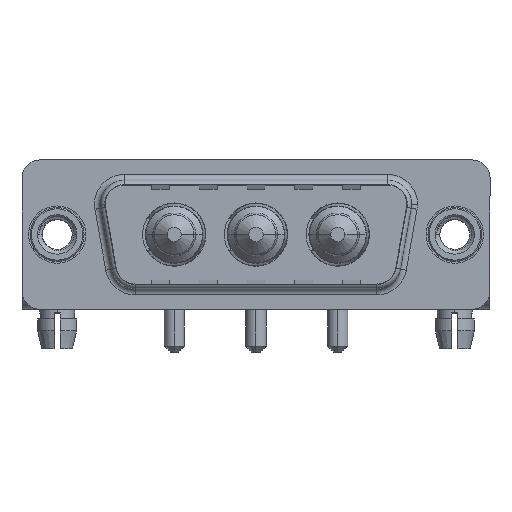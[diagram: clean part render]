
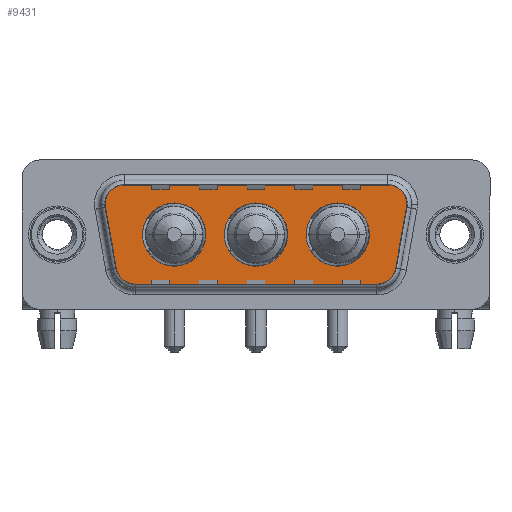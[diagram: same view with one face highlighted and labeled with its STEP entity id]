
A CAD part, top view. The second image highlights one B-rep face of the part: STEP entity #9431.
In plain terms, the highlighted planar face has unit normal (0, 0, 1).
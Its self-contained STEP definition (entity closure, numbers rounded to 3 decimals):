
#274 = VERTEX_POINT ( 'NONE', #9178 ) ;
#331 = FACE_BOUND ( 'NONE', #2962, .T. ) ;
#351 = EDGE_CURVE ( 'NONE', #10542, #8875, #3159, .T. ) ;
#378 = VERTEX_POINT ( 'NONE', #1753 ) ;
#496 = FACE_OUTER_BOUND ( 'NONE', #13904, .T. ) ;
#556 = CARTESIAN_POINT ( 'NONE',  ( 9.8, 0., 0. ) ) ;
#640 = CARTESIAN_POINT ( 'NONE',  ( 20.85, 0., 0. ) ) ;
#768 = ORIENTED_EDGE ( 'NONE', *, *, #11275, .T. ) ;
#896 = VERTEX_POINT ( 'NONE', #9669 ) ;
#897 = CARTESIAN_POINT ( 'NONE',  ( 3.441, 2.553, 0. ) ) ;
#939 = VERTEX_POINT ( 'NONE', #15259 ) ;
#1233 = VERTEX_POINT ( 'NONE', #13340 ) ;
#1234 = DIRECTION ( 'NONE',  ( 0., 0., 1. ) ) ;
#1381 = DIRECTION ( 'NONE',  ( -1., 0., 0. ) ) ;
#1605 = DIRECTION ( 'NONE',  ( 0., 0., 1. ) ) ;
#1616 = VECTOR ( 'NONE', #13439, 1000. ) ;
#1753 = CARTESIAN_POINT ( 'NONE',  ( 14., 0., 0. ) ) ;
#1831 = CARTESIAN_POINT ( 'NONE',  ( 23.5, 0., 0. ) ) ;
#1839 = DIRECTION ( 'NONE',  ( 0., 0., 1. ) ) ;
#1972 = CARTESIAN_POINT ( 'NONE',  ( 29.889, 2.9, 0. ) ) ;
#2001 = DIRECTION ( 'NONE',  ( -1., 0., 0. ) ) ;
#2114 = EDGE_CURVE ( 'NONE', #2596, #12028, #15450, .T. ) ;
#2161 = EDGE_LOOP ( 'NONE', ( #13981, #5495 ) ) ;
#2352 = DIRECTION ( 'NONE',  ( 1., 0., 0. ) ) ;
#2442 = CARTESIAN_POINT ( 'NONE',  ( 26.866, -4.9, 0. ) ) ;
#2596 = VERTEX_POINT ( 'NONE', #3486 ) ;
#2664 = DIRECTION ( 'NONE',  ( 0., 0., 1. ) ) ;
#2779 = ORIENTED_EDGE ( 'NONE', *, *, #13818, .F. ) ;
#2815 = FACE_BOUND ( 'NONE', #14606, .T. ) ;
#2962 = EDGE_LOOP ( 'NONE', ( #2779, #12236 ) ) ;
#2989 = CARTESIAN_POINT ( 'NONE',  ( 6.434, -4.9, 0. ) ) ;
#2990 = PLANE ( 'NONE',  #14527 ) ;
#3159 = CIRCLE ( 'NONE', #12820, 2.65 ) ;
#3203 = CARTESIAN_POINT ( 'NONE',  ( 27.889, 2.9, 0. ) ) ;
#3245 = CARTESIAN_POINT ( 'NONE',  ( 26.15, 0., 0. ) ) ;
#3306 = VERTEX_POINT ( 'NONE', #2442 ) ;
#3486 = CARTESIAN_POINT ( 'NONE',  ( 27.889, 4.9, 0. ) ) ;
#3535 = CIRCLE ( 'NONE', #10712, 2.65 ) ;
#3571 = DIRECTION ( 'NONE',  ( 1., 0., 0. ) ) ;
#3762 = CARTESIAN_POINT ( 'NONE',  ( 27.889, 2.9, 0. ) ) ;
#4209 = EDGE_CURVE ( 'NONE', #5974, #2596, #5596, .T. ) ;
#4340 = DIRECTION ( 'NONE',  ( 0., 0., 1. ) ) ;
#4402 = CARTESIAN_POINT ( 'NONE',  ( 12.45, 0., 0. ) ) ;
#4626 = EDGE_CURVE ( 'NONE', #378, #11603, #3535, .T. ) ;
#4787 = ORIENTED_EDGE ( 'NONE', *, *, #12151, .F. ) ;
#4800 = AXIS2_PLACEMENT_3D ( 'NONE', #3203, #1839, #2001 ) ;
#4841 = CIRCLE ( 'NONE', #7334, 2. ) ;
#5003 = LINE ( 'NONE', #897, #9470 ) ;
#5089 = CIRCLE ( 'NONE', #7308, 2.65 ) ;
#5100 = VERTEX_POINT ( 'NONE', #640 ) ;
#5268 = CARTESIAN_POINT ( 'NONE',  ( 16.65, 0., 0. ) ) ;
#5425 = ORIENTED_EDGE ( 'NONE', *, *, #4209, .T. ) ;
#5495 = ORIENTED_EDGE ( 'NONE', *, *, #8730, .F. ) ;
#5596 = CIRCLE ( 'NONE', #6151, 2. ) ;
#5646 = LINE ( 'NONE', #14955, #1616 ) ;
#5895 = CIRCLE ( 'NONE', #4800, 2. ) ;
#5974 = VERTEX_POINT ( 'NONE', #1972 ) ;
#6046 = DIRECTION ( 'NONE',  ( 1., 0., 0. ) ) ;
#6151 = AXIS2_PLACEMENT_3D ( 'NONE', #3762, #9035, #7483 ) ;
#6349 = EDGE_CURVE ( 'NONE', #1233, #3306, #10924, .T. ) ;
#6575 = CARTESIAN_POINT ( 'NONE',  ( 23.5, 0., 0. ) ) ;
#7308 = AXIS2_PLACEMENT_3D ( 'NONE', #1831, #12426, #6046 ) ;
#7334 = AXIS2_PLACEMENT_3D ( 'NONE', #10989, #4340, #1381 ) ;
#7359 = DIRECTION ( 'NONE',  ( -1., 0., 0. ) ) ;
#7436 = CARTESIAN_POINT ( 'NONE',  ( 5.411, 4.9, 0. ) ) ;
#7476 = CARTESIAN_POINT ( 'NONE',  ( 7.15, 0., 0. ) ) ;
#7483 = DIRECTION ( 'NONE',  ( -1., 0., 0. ) ) ;
#7925 = DIRECTION ( 'NONE',  ( 1., 0., 0. ) ) ;
#7970 = ORIENTED_EDGE ( 'NONE', *, *, #13523, .T. ) ;
#8233 = DIRECTION ( 'NONE',  ( 1., 0., 0. ) ) ;
#8308 = DIRECTION ( 'NONE',  ( 0., 0., 1. ) ) ;
#8381 = ORIENTED_EDGE ( 'NONE', *, *, #14727, .T. ) ;
#8510 = CIRCLE ( 'NONE', #9067, 2.65 ) ;
#8730 = EDGE_CURVE ( 'NONE', #8875, #10542, #8510, .T. ) ;
#8859 = ORIENTED_EDGE ( 'NONE', *, *, #2114, .T. ) ;
#8875 = VERTEX_POINT ( 'NONE', #7476 ) ;
#9035 = DIRECTION ( 'NONE',  ( 0., 0., 1. ) ) ;
#9067 = AXIS2_PLACEMENT_3D ( 'NONE', #14460, #2664, #7925 ) ;
#9178 = CARTESIAN_POINT ( 'NONE',  ( 3.441, 2.553, 0. ) ) ;
#9334 = VERTEX_POINT ( 'NONE', #15751 ) ;
#9413 = EDGE_CURVE ( 'NONE', #9334, #939, #5646, .T. ) ;
#9431 = ADVANCED_FACE ( 'NONE', ( #331, #2815, #10835, #496 ), #2990, .T. ) ;
#9470 = VECTOR ( 'NONE', #15270, 1000. ) ;
#9669 = CARTESIAN_POINT ( 'NONE',  ( 4.464, -3.247, 0. ) ) ;
#9840 = EDGE_CURVE ( 'NONE', #3306, #9334, #11967, .T. ) ;
#9943 = CARTESIAN_POINT ( 'NONE',  ( 5.411, 4.9, 0. ) ) ;
#10532 = EDGE_CURVE ( 'NONE', #12929, #5100, #5089, .T. ) ;
#10542 = VERTEX_POINT ( 'NONE', #4402 ) ;
#10658 = AXIS2_PLACEMENT_3D ( 'NONE', #6575, #12949, #14306 ) ;
#10677 = DIRECTION ( 'NONE',  ( 0., 0., 1. ) ) ;
#10712 = AXIS2_PLACEMENT_3D ( 'NONE', #12813, #14169, #3571 ) ;
#10757 = DIRECTION ( 'NONE',  ( 1., 0., 0. ) ) ;
#10835 = FACE_BOUND ( 'NONE', #2161, .T. ) ;
#10874 = AXIS2_PLACEMENT_3D ( 'NONE', #15986, #1605, #8233 ) ;
#10924 = LINE ( 'NONE', #2989, #14618 ) ;
#10989 = CARTESIAN_POINT ( 'NONE',  ( 6.434, -2.9, 0. ) ) ;
#11020 = ORIENTED_EDGE ( 'NONE', *, *, #6349, .T. ) ;
#11149 = AXIS2_PLACEMENT_3D ( 'NONE', #11643, #11561, #2352 ) ;
#11247 = VECTOR ( 'NONE', #7359, 1000. ) ;
#11275 = EDGE_CURVE ( 'NONE', #896, #1233, #4841, .T. ) ;
#11561 = DIRECTION ( 'NONE',  ( 0., 0., 1. ) ) ;
#11572 = ORIENTED_EDGE ( 'NONE', *, *, #9413, .T. ) ;
#11603 = VERTEX_POINT ( 'NONE', #16918 ) ;
#11643 = CARTESIAN_POINT ( 'NONE',  ( 5.411, 2.9, 0. ) ) ;
#11967 = CIRCLE ( 'NONE', #10874, 2. ) ;
#12028 = VERTEX_POINT ( 'NONE', #7436 ) ;
#12151 = EDGE_CURVE ( 'NONE', #5100, #12929, #13677, .T. ) ;
#12186 = DIRECTION ( 'NONE',  ( 1., 0., 0. ) ) ;
#12236 = ORIENTED_EDGE ( 'NONE', *, *, #4626, .F. ) ;
#12426 = DIRECTION ( 'NONE',  ( 0., 0., 1. ) ) ;
#12801 = CIRCLE ( 'NONE', #15529, 2.65 ) ;
#12813 = CARTESIAN_POINT ( 'NONE',  ( 16.65, 0., 0. ) ) ;
#12820 = AXIS2_PLACEMENT_3D ( 'NONE', #556, #8308, #12186 ) ;
#12929 = VERTEX_POINT ( 'NONE', #3245 ) ;
#12949 = DIRECTION ( 'NONE',  ( 0., 0., 1. ) ) ;
#13340 = CARTESIAN_POINT ( 'NONE',  ( 6.434, -4.9, 0. ) ) ;
#13345 = CARTESIAN_POINT ( 'NONE',  ( 26.866, -2.9, 0. ) ) ;
#13439 = DIRECTION ( 'NONE',  ( 0.174, 0.985, 0. ) ) ;
#13523 = EDGE_CURVE ( 'NONE', #274, #896, #5003, .T. ) ;
#13677 = CIRCLE ( 'NONE', #10658, 2.65 ) ;
#13818 = EDGE_CURVE ( 'NONE', #11603, #378, #12801, .T. ) ;
#13904 = EDGE_LOOP ( 'NONE', ( #16893, #11572, #8381, #5425, #8859, #16036, #7970, #768, #11020 ) ) ;
#13981 = ORIENTED_EDGE ( 'NONE', *, *, #351, .F. ) ;
#14169 = DIRECTION ( 'NONE',  ( 0., 0., 1. ) ) ;
#14306 = DIRECTION ( 'NONE',  ( 1., 0., 0. ) ) ;
#14460 = CARTESIAN_POINT ( 'NONE',  ( 9.8, 0., 0. ) ) ;
#14527 = AXIS2_PLACEMENT_3D ( 'NONE', #13345, #10677, #10757 ) ;
#14606 = EDGE_LOOP ( 'NONE', ( #16773, #4787 ) ) ;
#14618 = VECTOR ( 'NONE', #14871, 1000. ) ;
#14727 = EDGE_CURVE ( 'NONE', #939, #5974, #5895, .T. ) ;
#14871 = DIRECTION ( 'NONE',  ( 1., 0., 0. ) ) ;
#14888 = EDGE_CURVE ( 'NONE', #12028, #274, #16372, .T. ) ;
#14955 = CARTESIAN_POINT ( 'NONE',  ( 29.859, 2.553, 0. ) ) ;
#15259 = CARTESIAN_POINT ( 'NONE',  ( 29.859, 2.553, 0. ) ) ;
#15270 = DIRECTION ( 'NONE',  ( 0.174, -0.985, 0. ) ) ;
#15450 = LINE ( 'NONE', #9943, #11247 ) ;
#15529 = AXIS2_PLACEMENT_3D ( 'NONE', #5268, #1234, #15779 ) ;
#15751 = CARTESIAN_POINT ( 'NONE',  ( 28.836, -3.247, 0. ) ) ;
#15779 = DIRECTION ( 'NONE',  ( 1., 0., 0. ) ) ;
#15986 = CARTESIAN_POINT ( 'NONE',  ( 26.866, -2.9, 0. ) ) ;
#16036 = ORIENTED_EDGE ( 'NONE', *, *, #14888, .T. ) ;
#16372 = CIRCLE ( 'NONE', #11149, 2. ) ;
#16773 = ORIENTED_EDGE ( 'NONE', *, *, #10532, .F. ) ;
#16893 = ORIENTED_EDGE ( 'NONE', *, *, #9840, .T. ) ;
#16918 = CARTESIAN_POINT ( 'NONE',  ( 19.3, 0., 0. ) ) ;
